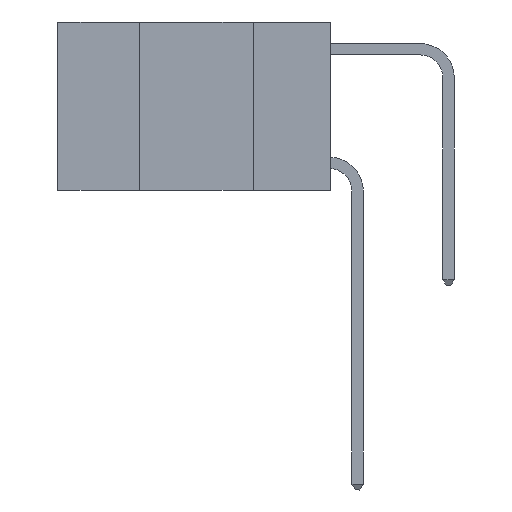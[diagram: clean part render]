
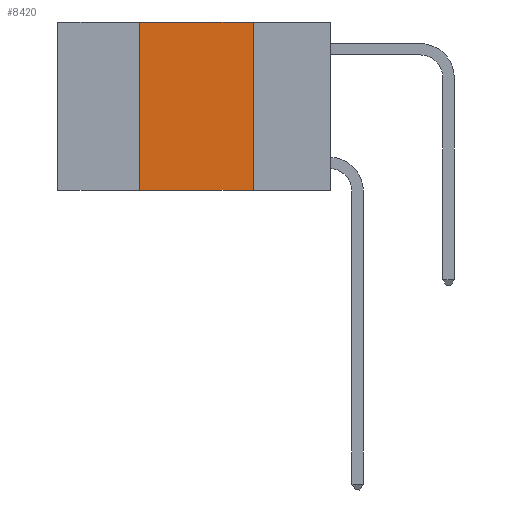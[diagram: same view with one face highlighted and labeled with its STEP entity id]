
A CAD part, left-side view. The second image highlights one B-rep face of the part: STEP entity #8420.
In plain terms, the highlighted planar face has unit normal (-1, 0, 0).
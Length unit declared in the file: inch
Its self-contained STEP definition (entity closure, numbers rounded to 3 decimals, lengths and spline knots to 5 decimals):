
#142 = DIRECTION ( 'NONE',  ( 0., 0., -1. ) ) ;
#770 = CARTESIAN_POINT ( 'NONE',  ( 0., 0.42, 0. ) ) ;
#1276 = CARTESIAN_POINT ( 'NONE',  ( 0., 0.17, 0. ) ) ;
#1349 = CARTESIAN_POINT ( 'NONE',  ( 0., 0.17, -0.37 ) ) ;
#1460 = EDGE_LOOP ( 'NONE', ( #3563, #4434, #7290, #13939 ) ) ;
#1523 = DIRECTION ( 'NONE',  ( 1., 0., 0. ) ) ;
#1708 = VECTOR ( 'NONE', #10259, 39.37008 ) ;
#1843 = LINE ( 'NONE', #6102, #11416 ) ;
#1915 = VERTEX_POINT ( 'NONE', #3164 ) ;
#2344 = PLANE ( 'NONE',  #6959 ) ;
#2421 = CARTESIAN_POINT ( 'NONE',  ( 0., 0.6, 0. ) ) ;
#2648 = VERTEX_POINT ( 'NONE', #13662 ) ;
#2707 = EDGE_CURVE ( 'NONE', #9920, #12490, #9989, .T. ) ;
#3034 = DIRECTION ( 'NONE',  ( 0., 0., 1. ) ) ;
#3164 = CARTESIAN_POINT ( 'NONE',  ( 0., 0.17, 0. ) ) ;
#3563 = ORIENTED_EDGE ( 'NONE', *, *, #12468, .F. ) ;
#3622 = FACE_OUTER_BOUND ( 'NONE', #1460, .T. ) ;
#4434 = ORIENTED_EDGE ( 'NONE', *, *, #8310, .F. ) ;
#4474 = VECTOR ( 'NONE', #3034, 39.37008 ) ;
#5754 = CARTESIAN_POINT ( 'NONE',  ( 0., 0.6, -0.37 ) ) ;
#5790 = DIRECTION ( 'NONE',  ( 0., 0., -1. ) ) ;
#6102 = CARTESIAN_POINT ( 'NONE',  ( 0., 0.6, 0. ) ) ;
#6281 = VECTOR ( 'NONE', #5790, 39.37008 ) ;
#6959 = AXIS2_PLACEMENT_3D ( 'NONE', #2421, #1523, #142 ) ;
#7289 = EDGE_CURVE ( 'NONE', #9920, #2648, #13087, .T. ) ;
#7290 = ORIENTED_EDGE ( 'NONE', *, *, #7289, .F. ) ;
#7438 = CARTESIAN_POINT ( 'NONE',  ( 0., 0.42, -0.37 ) ) ;
#8310 = EDGE_CURVE ( 'NONE', #2648, #1915, #1843, .T. ) ;
#8420 = ADVANCED_FACE ( 'NONE', ( #3622 ), #2344, .F. ) ;
#8635 = DIRECTION ( 'NONE',  ( 0., -1., 0. ) ) ;
#9920 = VERTEX_POINT ( 'NONE', #7438 ) ;
#9989 = LINE ( 'NONE', #5754, #1708 ) ;
#10259 = DIRECTION ( 'NONE',  ( 0., -1., 0. ) ) ;
#11397 = LINE ( 'NONE', #1276, #6281 ) ;
#11416 = VECTOR ( 'NONE', #8635, 39.37008 ) ;
#12468 = EDGE_CURVE ( 'NONE', #1915, #12490, #11397, .T. ) ;
#12490 = VERTEX_POINT ( 'NONE', #1349 ) ;
#13087 = LINE ( 'NONE', #770, #4474 ) ;
#13662 = CARTESIAN_POINT ( 'NONE',  ( 0., 0.42, 0. ) ) ;
#13939 = ORIENTED_EDGE ( 'NONE', *, *, #2707, .T. ) ;
